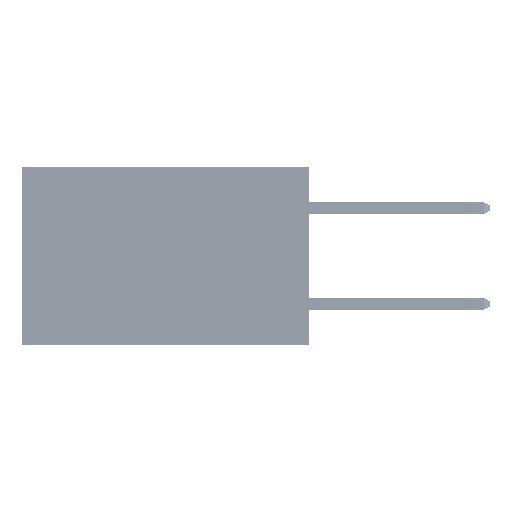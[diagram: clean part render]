
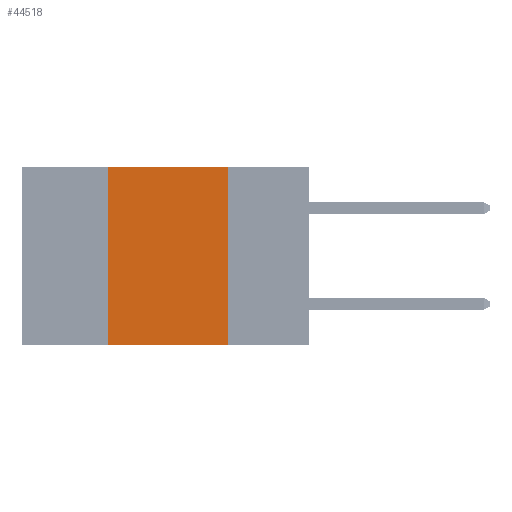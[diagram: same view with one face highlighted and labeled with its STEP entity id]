
A CAD part, left-side view. The second image highlights one B-rep face of the part: STEP entity #44518.
In plain terms, the highlighted planar face has unit normal (-1, 0, 0).
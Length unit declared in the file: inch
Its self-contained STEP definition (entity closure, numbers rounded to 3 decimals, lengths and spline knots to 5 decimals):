
#623 = CARTESIAN_POINT ( 'NONE',  ( 0., 0.17, 0. ) ) ;
#4994 = AXIS2_PLACEMENT_3D ( 'NONE', #34558, #12011, #11666 ) ;
#5391 = ORIENTED_EDGE ( 'NONE', *, *, #38431, .T. ) ;
#6862 = CARTESIAN_POINT ( 'NONE',  ( 0., 0.6, 0. ) ) ;
#6867 = LINE ( 'NONE', #623, #46189 ) ;
#8053 = VECTOR ( 'NONE', #33700, 39.37008 ) ;
#8104 = LINE ( 'NONE', #32154, #37328 ) ;
#10650 = EDGE_CURVE ( 'NONE', #35744, #18647, #36656, .T. ) ;
#11666 = DIRECTION ( 'NONE',  ( 0., 0., -1. ) ) ;
#12011 = DIRECTION ( 'NONE',  ( 1., 0., 0. ) ) ;
#14712 = EDGE_CURVE ( 'NONE', #27424, #35744, #45726, .T. ) ;
#18402 = CARTESIAN_POINT ( 'NONE',  ( 0., 0.42, 0. ) ) ;
#18647 = VERTEX_POINT ( 'NONE', #29989 ) ;
#19371 = VERTEX_POINT ( 'NONE', #34262 ) ;
#21260 = DIRECTION ( 'NONE',  ( 0., 0., 1. ) ) ;
#22931 = EDGE_LOOP ( 'NONE', ( #32971, #47494, #35877, #5391 ) ) ;
#27424 = VERTEX_POINT ( 'NONE', #46958 ) ;
#29989 = CARTESIAN_POINT ( 'NONE',  ( 0., 0.17, 0. ) ) ;
#30721 = PLANE ( 'NONE',  #4994 ) ;
#32154 = CARTESIAN_POINT ( 'NONE',  ( 0., 0.6, -0.37 ) ) ;
#32971 = ORIENTED_EDGE ( 'NONE', *, *, #38907, .F. ) ;
#33700 = DIRECTION ( 'NONE',  ( 0., -1., 0. ) ) ;
#34262 = CARTESIAN_POINT ( 'NONE',  ( 0., 0.17, -0.37 ) ) ;
#34558 = CARTESIAN_POINT ( 'NONE',  ( 0., 0.6, 0. ) ) ;
#35744 = VERTEX_POINT ( 'NONE', #18402 ) ;
#35877 = ORIENTED_EDGE ( 'NONE', *, *, #14712, .F. ) ;
#35951 = CARTESIAN_POINT ( 'NONE',  ( 0., 0.42, 0. ) ) ;
#36656 = LINE ( 'NONE', #6862, #8053 ) ;
#37328 = VECTOR ( 'NONE', #47448, 39.37008 ) ;
#38431 = EDGE_CURVE ( 'NONE', #27424, #19371, #8104, .T. ) ;
#38907 = EDGE_CURVE ( 'NONE', #18647, #19371, #6867, .T. ) ;
#41403 = FACE_OUTER_BOUND ( 'NONE', #22931, .T. ) ;
#44518 = ADVANCED_FACE ( 'NONE', ( #41403 ), #30721, .F. ) ;
#45726 = LINE ( 'NONE', #35951, #47509 ) ;
#45740 = DIRECTION ( 'NONE',  ( 0., 0., -1. ) ) ;
#46189 = VECTOR ( 'NONE', #45740, 39.37008 ) ;
#46958 = CARTESIAN_POINT ( 'NONE',  ( 0., 0.42, -0.37 ) ) ;
#47448 = DIRECTION ( 'NONE',  ( 0., -1., 0. ) ) ;
#47494 = ORIENTED_EDGE ( 'NONE', *, *, #10650, .F. ) ;
#47509 = VECTOR ( 'NONE', #21260, 39.37008 ) ;
